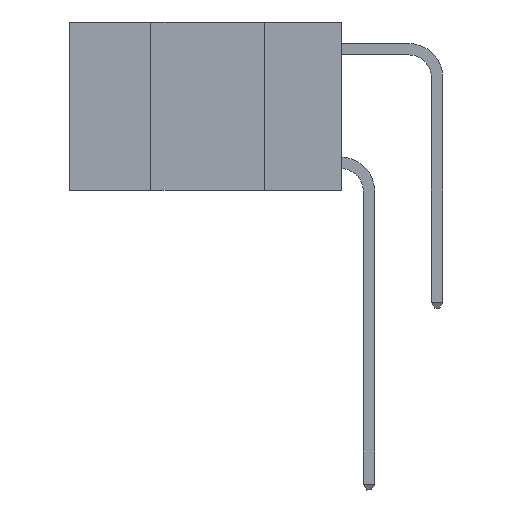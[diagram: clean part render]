
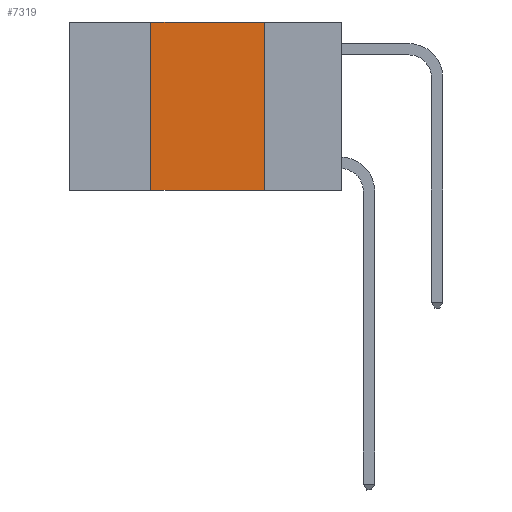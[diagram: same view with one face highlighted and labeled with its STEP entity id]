
A CAD part, left-side view. The second image highlights one B-rep face of the part: STEP entity #7319.
In plain terms, the highlighted planar face has unit normal (-1, 0, 0).
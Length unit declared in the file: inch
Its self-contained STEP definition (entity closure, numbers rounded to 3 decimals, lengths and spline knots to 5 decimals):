
#326 = CARTESIAN_POINT ( 'NONE',  ( 0., 0.42, 0. ) ) ;
#544 = CARTESIAN_POINT ( 'NONE',  ( 0., 0.6, 0. ) ) ;
#1503 = LINE ( 'NONE', #13620, #19450 ) ;
#2331 = CARTESIAN_POINT ( 'NONE',  ( 0., 0.6, 0. ) ) ;
#3688 = VERTEX_POINT ( 'NONE', #11301 ) ;
#3774 = CARTESIAN_POINT ( 'NONE',  ( 0., 0.6, -0.37 ) ) ;
#3957 = CARTESIAN_POINT ( 'NONE',  ( 0., 0.42, -0.37 ) ) ;
#4240 = PLANE ( 'NONE',  #5551 ) ;
#4927 = EDGE_LOOP ( 'NONE', ( #10725, #10973, #7944, #12694 ) ) ;
#5046 = EDGE_CURVE ( 'NONE', #9773, #9670, #1503, .T. ) ;
#5459 = DIRECTION ( 'NONE',  ( 0., -1., 0. ) ) ;
#5551 = AXIS2_PLACEMENT_3D ( 'NONE', #544, #12581, #15663 ) ;
#6820 = CARTESIAN_POINT ( 'NONE',  ( 0., 0.17, -0.37 ) ) ;
#6917 = DIRECTION ( 'NONE',  ( 0., -1., 0. ) ) ;
#7129 = EDGE_CURVE ( 'NONE', #7148, #9670, #17398, .T. ) ;
#7148 = VERTEX_POINT ( 'NONE', #3957 ) ;
#7319 = ADVANCED_FACE ( 'NONE', ( #19369 ), #4240, .F. ) ;
#7912 = LINE ( 'NONE', #326, #17934 ) ;
#7944 = ORIENTED_EDGE ( 'NONE', *, *, #16188, .F. ) ;
#9646 = VECTOR ( 'NONE', #5459, 39.37008 ) ;
#9670 = VERTEX_POINT ( 'NONE', #6820 ) ;
#9773 = VERTEX_POINT ( 'NONE', #19444 ) ;
#9899 = LINE ( 'NONE', #2331, #19583 ) ;
#10725 = ORIENTED_EDGE ( 'NONE', *, *, #5046, .F. ) ;
#10973 = ORIENTED_EDGE ( 'NONE', *, *, #18372, .F. ) ;
#11301 = CARTESIAN_POINT ( 'NONE',  ( 0., 0.42, 0. ) ) ;
#12581 = DIRECTION ( 'NONE',  ( 1., 0., 0. ) ) ;
#12694 = ORIENTED_EDGE ( 'NONE', *, *, #7129, .T. ) ;
#13620 = CARTESIAN_POINT ( 'NONE',  ( 0., 0.17, 0. ) ) ;
#14825 = DIRECTION ( 'NONE',  ( 0., 0., -1. ) ) ;
#15456 = DIRECTION ( 'NONE',  ( 0., 0., 1. ) ) ;
#15663 = DIRECTION ( 'NONE',  ( 0., 0., -1. ) ) ;
#16188 = EDGE_CURVE ( 'NONE', #7148, #3688, #7912, .T. ) ;
#17398 = LINE ( 'NONE', #3774, #9646 ) ;
#17934 = VECTOR ( 'NONE', #15456, 39.37008 ) ;
#18372 = EDGE_CURVE ( 'NONE', #3688, #9773, #9899, .T. ) ;
#19369 = FACE_OUTER_BOUND ( 'NONE', #4927, .T. ) ;
#19444 = CARTESIAN_POINT ( 'NONE',  ( 0., 0.17, 0. ) ) ;
#19450 = VECTOR ( 'NONE', #14825, 39.37008 ) ;
#19583 = VECTOR ( 'NONE', #6917, 39.37008 ) ;
